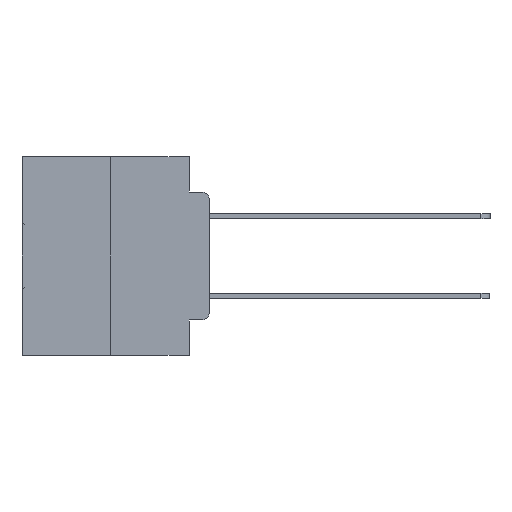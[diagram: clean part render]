
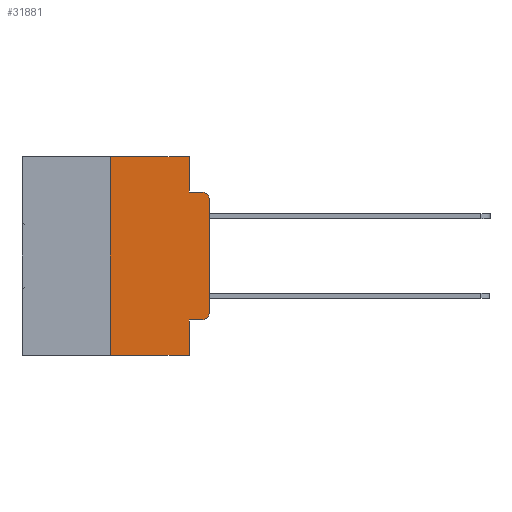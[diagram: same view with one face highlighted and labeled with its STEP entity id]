
A CAD part, left-side view. The second image highlights one B-rep face of the part: STEP entity #31881.
In plain terms, the highlighted planar face has unit normal (-1, 0, 0).
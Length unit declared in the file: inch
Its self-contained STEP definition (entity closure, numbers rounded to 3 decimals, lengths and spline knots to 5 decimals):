
#126 = DIRECTION ( 'NONE',  ( 0., 0., -1. ) ) ;
#309 = VERTEX_POINT ( 'NONE', #24227 ) ;
#1107 = ORIENTED_EDGE ( 'NONE', *, *, #19138, .T. ) ;
#2865 = DIRECTION ( 'NONE',  ( 0., -1., 0. ) ) ;
#3104 = LINE ( 'NONE', #23596, #23120 ) ;
#5368 = LINE ( 'NONE', #25766, #33182 ) ;
#5530 = CARTESIAN_POINT ( 'NONE',  ( 0., 0.051, 0. ) ) ;
#5579 = FACE_OUTER_BOUND ( 'NONE', #7536, .T. ) ;
#6209 = ORIENTED_EDGE ( 'NONE', *, *, #13591, .F. ) ;
#6491 = CARTESIAN_POINT ( 'NONE',  ( 0., 0.02, -0.3915 ) ) ;
#6576 = CARTESIAN_POINT ( 'NONE',  ( 0., 0.02, -0.4115 ) ) ;
#6705 = DIRECTION ( 'NONE',  ( 0., -1., 0. ) ) ;
#6821 = LINE ( 'NONE', #32643, #20413 ) ;
#7536 = EDGE_LOOP ( 'NONE', ( #10227, #30601, #29925, #9991, #6209, #15561, #1107, #17664, #15034, #16049 ) ) ;
#7543 = LINE ( 'NONE', #29444, #14005 ) ;
#7615 = CIRCLE ( 'NONE', #30849, 0.02 ) ;
#7625 = EDGE_CURVE ( 'NONE', #18696, #19330, #22668, .T. ) ;
#7762 = LINE ( 'NONE', #20248, #14235 ) ;
#8782 = EDGE_CURVE ( 'NONE', #31467, #34739, #7762, .T. ) ;
#9287 = DIRECTION ( 'NONE',  ( 0., 0., -1. ) ) ;
#9436 = CARTESIAN_POINT ( 'NONE',  ( 0., 0.02, -0.1085 ) ) ;
#9991 = ORIENTED_EDGE ( 'NONE', *, *, #19927, .F. ) ;
#10227 = ORIENTED_EDGE ( 'NONE', *, *, #30515, .T. ) ;
#10954 = VECTOR ( 'NONE', #11059, 39.37008 ) ;
#11059 = DIRECTION ( 'NONE',  ( 0., 0., -1. ) ) ;
#11312 = CARTESIAN_POINT ( 'NONE',  ( 0., 0., -0.3915 ) ) ;
#12199 = DIRECTION ( 'NONE',  ( 0., 0., -1. ) ) ;
#12434 = DIRECTION ( 'NONE',  ( 0., -1., 0. ) ) ;
#12642 = EDGE_CURVE ( 'NONE', #33747, #34739, #7615, .T. ) ;
#12942 = DIRECTION ( 'NONE',  ( 0., 0., 1. ) ) ;
#13591 = EDGE_CURVE ( 'NONE', #19330, #34941, #7543, .T. ) ;
#14005 = VECTOR ( 'NONE', #26764, 39.37008 ) ;
#14235 = VECTOR ( 'NONE', #6705, 39.37008 ) ;
#14511 = AXIS2_PLACEMENT_3D ( 'NONE', #6491, #25404, #9287 ) ;
#15034 = ORIENTED_EDGE ( 'NONE', *, *, #32573, .T. ) ;
#15100 = VECTOR ( 'NONE', #12942, 39.37008 ) ;
#15561 = ORIENTED_EDGE ( 'NONE', *, *, #7625, .F. ) ;
#16049 = ORIENTED_EDGE ( 'NONE', *, *, #21402, .T. ) ;
#16605 = VERTEX_POINT ( 'NONE', #11312 ) ;
#16646 = DIRECTION ( 'NONE',  ( 1., 0., 0. ) ) ;
#17664 = ORIENTED_EDGE ( 'NONE', *, *, #20089, .F. ) ;
#18128 = LINE ( 'NONE', #19082, #10954 ) ;
#18249 = CARTESIAN_POINT ( 'NONE',  ( 0., 0., 0. ) ) ;
#18696 = VERTEX_POINT ( 'NONE', #21222 ) ;
#18863 = CIRCLE ( 'NONE', #14511, 0.02 ) ;
#19082 = CARTESIAN_POINT ( 'NONE',  ( 0., 0.051, 0. ) ) ;
#19138 = EDGE_CURVE ( 'NONE', #18696, #34083, #5368, .T. ) ;
#19330 = VERTEX_POINT ( 'NONE', #29367 ) ;
#19927 = EDGE_CURVE ( 'NONE', #34941, #31467, #3104, .T. ) ;
#20089 = EDGE_CURVE ( 'NONE', #309, #34083, #18128, .T. ) ;
#20248 = CARTESIAN_POINT ( 'NONE',  ( 0., 0.051, -0.0885 ) ) ;
#20413 = VECTOR ( 'NONE', #2865, 39.37008 ) ;
#21222 = CARTESIAN_POINT ( 'NONE',  ( 0., 0.25, -0.5 ) ) ;
#21402 = EDGE_CURVE ( 'NONE', #33937, #16605, #18863, .T. ) ;
#22176 = LINE ( 'NONE', #18249, #15100 ) ;
#22668 = LINE ( 'NONE', #31131, #28934 ) ;
#23120 = VECTOR ( 'NONE', #26424, 39.37008 ) ;
#23465 = CARTESIAN_POINT ( 'NONE',  ( 0., 0.051, -0.5 ) ) ;
#23596 = CARTESIAN_POINT ( 'NONE',  ( 0., 0.051, 0. ) ) ;
#24227 = CARTESIAN_POINT ( 'NONE',  ( 0., 0.051, -0.4115 ) ) ;
#25404 = DIRECTION ( 'NONE',  ( -1., 0., 0. ) ) ;
#25766 = CARTESIAN_POINT ( 'NONE',  ( 0., 0.473, -0.5 ) ) ;
#26424 = DIRECTION ( 'NONE',  ( 0., 0., -1. ) ) ;
#26764 = DIRECTION ( 'NONE',  ( 0., -1., 0. ) ) ;
#28246 = DIRECTION ( 'NONE',  ( -1., 0., 0. ) ) ;
#28934 = VECTOR ( 'NONE', #33806, 39.37008 ) ;
#29367 = CARTESIAN_POINT ( 'NONE',  ( 0., 0.25, 0. ) ) ;
#29444 = CARTESIAN_POINT ( 'NONE',  ( 0., 0.473, 0. ) ) ;
#29925 = ORIENTED_EDGE ( 'NONE', *, *, #8782, .F. ) ;
#29933 = PLANE ( 'NONE',  #34027 ) ;
#30515 = EDGE_CURVE ( 'NONE', #16605, #33747, #22176, .T. ) ;
#30601 = ORIENTED_EDGE ( 'NONE', *, *, #12642, .T. ) ;
#30849 = AXIS2_PLACEMENT_3D ( 'NONE', #9436, #28246, #12199 ) ;
#31131 = CARTESIAN_POINT ( 'NONE',  ( 0., 0.25, 0. ) ) ;
#31467 = VERTEX_POINT ( 'NONE', #33319 ) ;
#31568 = CARTESIAN_POINT ( 'NONE',  ( 0., 0.02, -0.0885 ) ) ;
#31881 = ADVANCED_FACE ( 'NONE', ( #5579 ), #29933, .F. ) ;
#32573 = EDGE_CURVE ( 'NONE', #309, #33937, #6821, .T. ) ;
#32576 = CARTESIAN_POINT ( 'NONE',  ( 0., 0.473, 0. ) ) ;
#32643 = CARTESIAN_POINT ( 'NONE',  ( 0., 0.051, -0.4115 ) ) ;
#33182 = VECTOR ( 'NONE', #12434, 39.37008 ) ;
#33319 = CARTESIAN_POINT ( 'NONE',  ( 0., 0.051, -0.0885 ) ) ;
#33747 = VERTEX_POINT ( 'NONE', #34641 ) ;
#33806 = DIRECTION ( 'NONE',  ( 0., 0., 1. ) ) ;
#33937 = VERTEX_POINT ( 'NONE', #6576 ) ;
#34027 = AXIS2_PLACEMENT_3D ( 'NONE', #32576, #16646, #126 ) ;
#34083 = VERTEX_POINT ( 'NONE', #23465 ) ;
#34641 = CARTESIAN_POINT ( 'NONE',  ( 0., 0., -0.1085 ) ) ;
#34739 = VERTEX_POINT ( 'NONE', #31568 ) ;
#34941 = VERTEX_POINT ( 'NONE', #5530 ) ;
